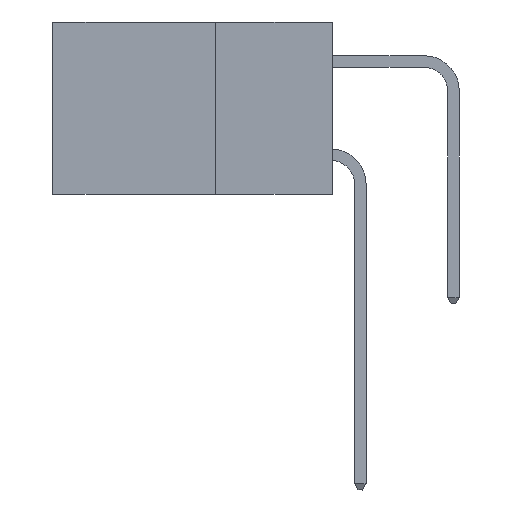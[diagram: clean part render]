
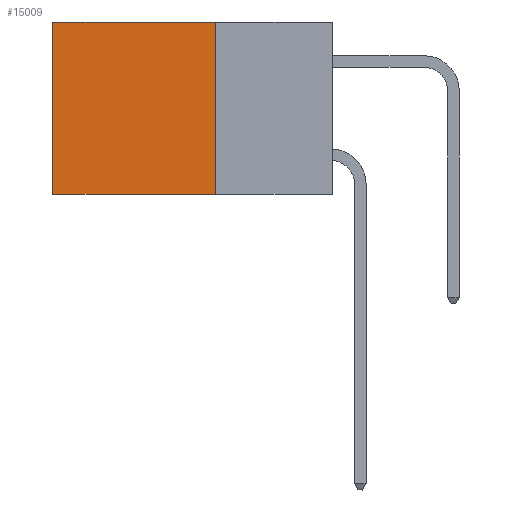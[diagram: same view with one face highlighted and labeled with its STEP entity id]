
A CAD part, left-side view. The second image highlights one B-rep face of the part: STEP entity #15009.
In plain terms, the highlighted planar face has unit normal (-1, 0, 0).
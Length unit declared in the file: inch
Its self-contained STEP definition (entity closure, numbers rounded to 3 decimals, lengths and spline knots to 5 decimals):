
#225 = LINE ( 'NONE', #9007, #15451 ) ;
#824 = VERTEX_POINT ( 'NONE', #8610 ) ;
#1116 = LINE ( 'NONE', #16837, #14546 ) ;
#1514 = EDGE_LOOP ( 'NONE', ( #5567, #6055, #17480, #9033 ) ) ;
#1966 = AXIS2_PLACEMENT_3D ( 'NONE', #17879, #6520, #6225 ) ;
#2116 = CARTESIAN_POINT ( 'NONE',  ( 0.2615, 0.6, 0. ) ) ;
#3468 = FACE_OUTER_BOUND ( 'NONE', #1514, .T. ) ;
#3715 = DIRECTION ( 'NONE',  ( 0., 0., -1. ) ) ;
#3861 = VERTEX_POINT ( 'NONE', #6835 ) ;
#4137 = DIRECTION ( 'NONE',  ( 0., 1., 0. ) ) ;
#5567 = ORIENTED_EDGE ( 'NONE', *, *, #7888, .T. ) ;
#5783 = VERTEX_POINT ( 'NONE', #2116 ) ;
#5813 = LINE ( 'NONE', #7333, #11786 ) ;
#6055 = ORIENTED_EDGE ( 'NONE', *, *, #12190, .F. ) ;
#6075 = CARTESIAN_POINT ( 'NONE',  ( 0.2615, 0.25, 0. ) ) ;
#6225 = DIRECTION ( 'NONE',  ( 0., 0., -1. ) ) ;
#6308 = EDGE_CURVE ( 'NONE', #12215, #5783, #5813, .T. ) ;
#6520 = DIRECTION ( 'NONE',  ( 1., 0., 0. ) ) ;
#6536 = EDGE_CURVE ( 'NONE', #12215, #824, #1116, .T. ) ;
#6835 = CARTESIAN_POINT ( 'NONE',  ( 0.2615, 0.6, -0.37 ) ) ;
#7333 = CARTESIAN_POINT ( 'NONE',  ( 0.2615, 0.25, 0. ) ) ;
#7888 = EDGE_CURVE ( 'NONE', #5783, #3861, #225, .T. ) ;
#8610 = CARTESIAN_POINT ( 'NONE',  ( 0.2615, 0.25, -0.37 ) ) ;
#9007 = CARTESIAN_POINT ( 'NONE',  ( 0.2615, 0.6, -0.37 ) ) ;
#9033 = ORIENTED_EDGE ( 'NONE', *, *, #6308, .T. ) ;
#10557 = DIRECTION ( 'NONE',  ( 0., 0., -1. ) ) ;
#11786 = VECTOR ( 'NONE', #4137, 39.37008 ) ;
#12190 = EDGE_CURVE ( 'NONE', #824, #3861, #17563, .T. ) ;
#12215 = VERTEX_POINT ( 'NONE', #6075 ) ;
#13289 = DIRECTION ( 'NONE',  ( 0., 1., 0. ) ) ;
#14546 = VECTOR ( 'NONE', #3715, 39.37008 ) ;
#15009 = ADVANCED_FACE ( 'NONE', ( #3468 ), #16481, .F. ) ;
#15451 = VECTOR ( 'NONE', #10557, 39.37008 ) ;
#16481 = PLANE ( 'NONE',  #1966 ) ;
#16542 = CARTESIAN_POINT ( 'NONE',  ( 0.2615, 0.25, -0.37 ) ) ;
#16837 = CARTESIAN_POINT ( 'NONE',  ( 0.2615, 0.25, -0.37 ) ) ;
#17480 = ORIENTED_EDGE ( 'NONE', *, *, #6536, .F. ) ;
#17563 = LINE ( 'NONE', #16542, #17953 ) ;
#17879 = CARTESIAN_POINT ( 'NONE',  ( 0.2615, 0.25, -0.37 ) ) ;
#17953 = VECTOR ( 'NONE', #13289, 39.37008 ) ;
